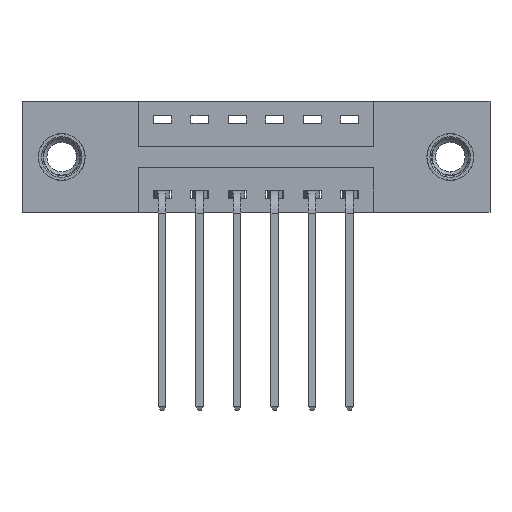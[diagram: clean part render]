
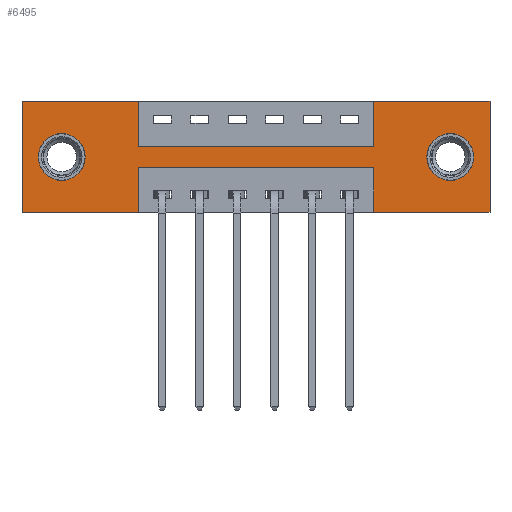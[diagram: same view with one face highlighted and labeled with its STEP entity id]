
A CAD part, front view. The second image highlights one B-rep face of the part: STEP entity #6495.
In plain terms, the highlighted planar face has unit normal (0, -1, 0).
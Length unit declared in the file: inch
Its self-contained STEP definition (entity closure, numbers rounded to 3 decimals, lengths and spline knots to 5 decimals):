
#119 = VERTEX_POINT ( 'NONE', #9369 ) ;
#244 = ORIENTED_EDGE ( 'NONE', *, *, #2837, .F. ) ;
#289 = VERTEX_POINT ( 'NONE', #1425 ) ;
#305 = DIRECTION ( 'NONE',  ( 1., 0., 0. ) ) ;
#339 = ORIENTED_EDGE ( 'NONE', *, *, #5300, .T. ) ;
#354 = VERTEX_POINT ( 'NONE', #7868 ) ;
#388 = ORIENTED_EDGE ( 'NONE', *, *, #5562, .F. ) ;
#436 = CIRCLE ( 'NONE', #3258, 0.078 ) ;
#577 = EDGE_CURVE ( 'NONE', #3117, #4924, #2016, .T. ) ;
#773 = DIRECTION ( 'NONE',  ( 0., 0., -1. ) ) ;
#817 = FACE_BOUND ( 'NONE', #4239, .T. ) ;
#1013 = CARTESIAN_POINT ( 'NONE',  ( 0.1325, 0., -0.185 ) ) ;
#1054 = LINE ( 'NONE', #1777, #3829 ) ;
#1078 = VERTEX_POINT ( 'NONE', #4053 ) ;
#1113 = ORIENTED_EDGE ( 'NONE', *, *, #7208, .F. ) ;
#1242 = DIRECTION ( 'NONE',  ( -1., 0., 0. ) ) ;
#1342 = CARTESIAN_POINT ( 'NONE',  ( 0., 0., -0.37 ) ) ;
#1425 = CARTESIAN_POINT ( 'NONE',  ( 1.4275, 0., -0.107 ) ) ;
#1459 = CARTESIAN_POINT ( 'NONE',  ( 0.3875, 0., -0.37 ) ) ;
#1561 = LINE ( 'NONE', #4471, #3824 ) ;
#1585 = CARTESIAN_POINT ( 'NONE',  ( 0., 0., -0.37 ) ) ;
#1641 = VERTEX_POINT ( 'NONE', #1970 ) ;
#1662 = CARTESIAN_POINT ( 'NONE',  ( 0.1325, 0., -0.107 ) ) ;
#1675 = VECTOR ( 'NONE', #4566, 39.37008 ) ;
#1766 = VERTEX_POINT ( 'NONE', #1342 ) ;
#1777 = CARTESIAN_POINT ( 'NONE',  ( 0.3875, 0., -0.15 ) ) ;
#1821 = EDGE_CURVE ( 'NONE', #4924, #3598, #8453, .T. ) ;
#1834 = EDGE_CURVE ( 'NONE', #4633, #8227, #3864, .T. ) ;
#1918 = LINE ( 'NONE', #3395, #2780 ) ;
#1936 = CARTESIAN_POINT ( 'NONE',  ( 1.1725, 0., 0. ) ) ;
#1958 = CARTESIAN_POINT ( 'NONE',  ( 0., 0., 0. ) ) ;
#1970 = CARTESIAN_POINT ( 'NONE',  ( 0., 0., 0. ) ) ;
#2016 = LINE ( 'NONE', #5042, #7048 ) ;
#2060 = DIRECTION ( 'NONE',  ( 0., 0., 1. ) ) ;
#2095 = LINE ( 'NONE', #5868, #7559 ) ;
#2136 = ORIENTED_EDGE ( 'NONE', *, *, #8696, .F. ) ;
#2138 = AXIS2_PLACEMENT_3D ( 'NONE', #5143, #8930, #2060 ) ;
#2307 = AXIS2_PLACEMENT_3D ( 'NONE', #3176, #3331, #9502 ) ;
#2527 = EDGE_CURVE ( 'NONE', #289, #7396, #436, .T. ) ;
#2536 = VERTEX_POINT ( 'NONE', #6558 ) ;
#2598 = VECTOR ( 'NONE', #4609, 39.37008 ) ;
#2644 = ORIENTED_EDGE ( 'NONE', *, *, #3797, .F. ) ;
#2721 = CARTESIAN_POINT ( 'NONE',  ( 1.4275, 0., -0.263 ) ) ;
#2749 = DIRECTION ( 'NONE',  ( 0., 1., 0. ) ) ;
#2780 = VECTOR ( 'NONE', #1242, 39.37008 ) ;
#2837 = EDGE_CURVE ( 'NONE', #4571, #354, #8273, .T. ) ;
#2839 = EDGE_CURVE ( 'NONE', #9498, #2536, #1561, .T. ) ;
#2979 = CARTESIAN_POINT ( 'NONE',  ( 0., 0., 0. ) ) ;
#3036 = LINE ( 'NONE', #6058, #1675 ) ;
#3117 = VERTEX_POINT ( 'NONE', #4995 ) ;
#3159 = ORIENTED_EDGE ( 'NONE', *, *, #2839, .F. ) ;
#3176 = CARTESIAN_POINT ( 'NONE',  ( 1.4275, 0., -0.185 ) ) ;
#3240 = CARTESIAN_POINT ( 'NONE',  ( 0., 0., -0.37 ) ) ;
#3258 = AXIS2_PLACEMENT_3D ( 'NONE', #6510, #2749, #4257 ) ;
#3331 = DIRECTION ( 'NONE',  ( 0., 1., 0. ) ) ;
#3371 = EDGE_CURVE ( 'NONE', #8227, #4633, #8661, .T. ) ;
#3395 = CARTESIAN_POINT ( 'NONE',  ( 0.3875, 0., -0.22 ) ) ;
#3598 = VERTEX_POINT ( 'NONE', #5792 ) ;
#3656 = ORIENTED_EDGE ( 'NONE', *, *, #4892, .F. ) ;
#3737 = DIRECTION ( 'NONE',  ( -1., 0., 0. ) ) ;
#3797 = EDGE_CURVE ( 'NONE', #354, #1766, #7009, .T. ) ;
#3824 = VECTOR ( 'NONE', #7544, 39.37008 ) ;
#3829 = VECTOR ( 'NONE', #305, 39.37008 ) ;
#3864 = CIRCLE ( 'NONE', #2138, 0.078 ) ;
#3934 = DIRECTION ( 'NONE',  ( 0., -1., 0. ) ) ;
#4053 = CARTESIAN_POINT ( 'NONE',  ( 1.1725, 0., -0.15 ) ) ;
#4239 = EDGE_LOOP ( 'NONE', ( #5445, #339 ) ) ;
#4257 = DIRECTION ( 'NONE',  ( 0., 0., -1. ) ) ;
#4288 = DIRECTION ( 'NONE',  ( 0., 1., 0. ) ) ;
#4471 = CARTESIAN_POINT ( 'NONE',  ( 0.3875, 0., 0. ) ) ;
#4515 = CARTESIAN_POINT ( 'NONE',  ( 0.3875, 0., 0. ) ) ;
#4566 = DIRECTION ( 'NONE',  ( 1., 0., 0. ) ) ;
#4570 = ORIENTED_EDGE ( 'NONE', *, *, #9165, .F. ) ;
#4571 = VERTEX_POINT ( 'NONE', #8042 ) ;
#4609 = DIRECTION ( 'NONE',  ( -1., 0., 0. ) ) ;
#4633 = VERTEX_POINT ( 'NONE', #8282 ) ;
#4685 = FACE_BOUND ( 'NONE', #7534, .T. ) ;
#4726 = ORIENTED_EDGE ( 'NONE', *, *, #3371, .T. ) ;
#4728 = VERTEX_POINT ( 'NONE', #6281 ) ;
#4892 = EDGE_CURVE ( 'NONE', #3598, #119, #2095, .T. ) ;
#4924 = VERTEX_POINT ( 'NONE', #8919 ) ;
#4950 = AXIS2_PLACEMENT_3D ( 'NONE', #1013, #4288, #9387 ) ;
#4995 = CARTESIAN_POINT ( 'NONE',  ( 1.56, 0., 0. ) ) ;
#5009 = ORIENTED_EDGE ( 'NONE', *, *, #7275, .F. ) ;
#5032 = LINE ( 'NONE', #1958, #5769 ) ;
#5042 = CARTESIAN_POINT ( 'NONE',  ( 1.56, 0., 0. ) ) ;
#5143 = CARTESIAN_POINT ( 'NONE',  ( 0.1325, 0., -0.185 ) ) ;
#5300 = EDGE_CURVE ( 'NONE', #7396, #289, #9488, .T. ) ;
#5445 = ORIENTED_EDGE ( 'NONE', *, *, #2527, .T. ) ;
#5562 = EDGE_CURVE ( 'NONE', #4728, #3117, #3036, .T. ) ;
#5769 = VECTOR ( 'NONE', #7236, 39.37008 ) ;
#5792 = CARTESIAN_POINT ( 'NONE',  ( 1.1725, 0., -0.37 ) ) ;
#5868 = CARTESIAN_POINT ( 'NONE',  ( 1.1725, 0., -0.37 ) ) ;
#5885 = EDGE_LOOP ( 'NONE', ( #244, #4570, #3656, #8725, #5890, #388, #1113, #2136, #3159, #6777, #5009, #2644 ) ) ;
#5890 = ORIENTED_EDGE ( 'NONE', *, *, #577, .F. ) ;
#6058 = CARTESIAN_POINT ( 'NONE',  ( 0., 0., 0. ) ) ;
#6062 = VECTOR ( 'NONE', #7362, 39.37008 ) ;
#6131 = DIRECTION ( 'NONE',  ( 0., 0., -1. ) ) ;
#6281 = CARTESIAN_POINT ( 'NONE',  ( 1.1725, 0., 0. ) ) ;
#6495 = ADVANCED_FACE ( 'NONE', ( #817, #4685, #8618 ), #7657, .T. ) ;
#6510 = CARTESIAN_POINT ( 'NONE',  ( 1.4275, 0., -0.185 ) ) ;
#6558 = CARTESIAN_POINT ( 'NONE',  ( 0.3875, 0., -0.15 ) ) ;
#6777 = ORIENTED_EDGE ( 'NONE', *, *, #9341, .F. ) ;
#7009 = LINE ( 'NONE', #9201, #2598 ) ;
#7048 = VECTOR ( 'NONE', #8131, 39.37008 ) ;
#7111 = DIRECTION ( 'NONE',  ( 0., 0., 1. ) ) ;
#7208 = EDGE_CURVE ( 'NONE', #1078, #4728, #8643, .T. ) ;
#7236 = DIRECTION ( 'NONE',  ( 1., 0., 0. ) ) ;
#7275 = EDGE_CURVE ( 'NONE', #1766, #1641, #9087, .T. ) ;
#7362 = DIRECTION ( 'NONE',  ( 0., 0., 1. ) ) ;
#7396 = VERTEX_POINT ( 'NONE', #2721 ) ;
#7534 = EDGE_LOOP ( 'NONE', ( #4726, #9376 ) ) ;
#7544 = DIRECTION ( 'NONE',  ( 0., 0., -1. ) ) ;
#7559 = VECTOR ( 'NONE', #9108, 39.37008 ) ;
#7657 = PLANE ( 'NONE',  #9427 ) ;
#7868 = CARTESIAN_POINT ( 'NONE',  ( 0.3875, 0., -0.37 ) ) ;
#8042 = CARTESIAN_POINT ( 'NONE',  ( 0.3875, 0., -0.22 ) ) ;
#8131 = DIRECTION ( 'NONE',  ( 0., 0., -1. ) ) ;
#8185 = VECTOR ( 'NONE', #773, 39.37008 ) ;
#8223 = VECTOR ( 'NONE', #3737, 39.37008 ) ;
#8227 = VERTEX_POINT ( 'NONE', #1662 ) ;
#8273 = LINE ( 'NONE', #1459, #8185 ) ;
#8282 = CARTESIAN_POINT ( 'NONE',  ( 0.1325, 0., -0.263 ) ) ;
#8453 = LINE ( 'NONE', #1585, #8223 ) ;
#8618 = FACE_OUTER_BOUND ( 'NONE', #5885, .T. ) ;
#8643 = LINE ( 'NONE', #1936, #9141 ) ;
#8661 = CIRCLE ( 'NONE', #4950, 0.078 ) ;
#8696 = EDGE_CURVE ( 'NONE', #2536, #1078, #1054, .T. ) ;
#8725 = ORIENTED_EDGE ( 'NONE', *, *, #1821, .F. ) ;
#8919 = CARTESIAN_POINT ( 'NONE',  ( 1.56, 0., -0.37 ) ) ;
#8930 = DIRECTION ( 'NONE',  ( 0., 1., 0. ) ) ;
#9087 = LINE ( 'NONE', #2979, #6062 ) ;
#9108 = DIRECTION ( 'NONE',  ( 0., 0., 1. ) ) ;
#9141 = VECTOR ( 'NONE', #7111, 39.37008 ) ;
#9165 = EDGE_CURVE ( 'NONE', #119, #4571, #1918, .T. ) ;
#9201 = CARTESIAN_POINT ( 'NONE',  ( 0., 0., -0.37 ) ) ;
#9341 = EDGE_CURVE ( 'NONE', #1641, #9498, #5032, .T. ) ;
#9369 = CARTESIAN_POINT ( 'NONE',  ( 1.1725, 0., -0.22 ) ) ;
#9376 = ORIENTED_EDGE ( 'NONE', *, *, #1834, .T. ) ;
#9387 = DIRECTION ( 'NONE',  ( 0., 0., 1. ) ) ;
#9427 = AXIS2_PLACEMENT_3D ( 'NONE', #3240, #3934, #6131 ) ;
#9488 = CIRCLE ( 'NONE', #2307, 0.078 ) ;
#9498 = VERTEX_POINT ( 'NONE', #4515 ) ;
#9502 = DIRECTION ( 'NONE',  ( 0., 0., -1. ) ) ;
